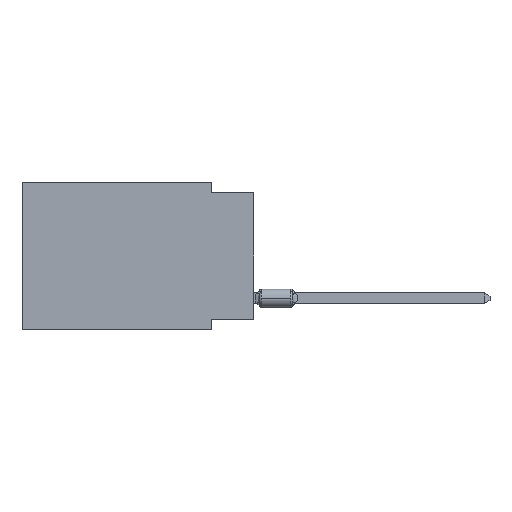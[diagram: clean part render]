
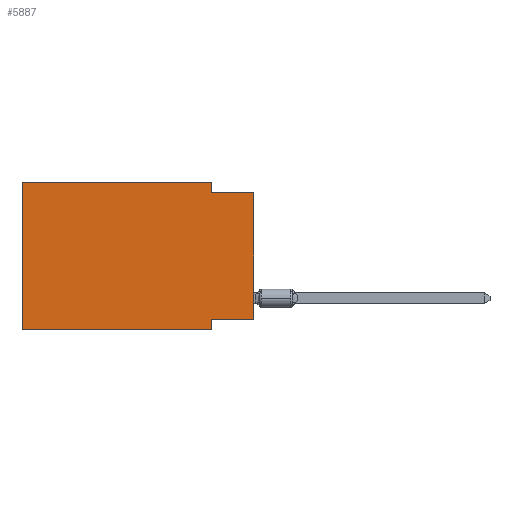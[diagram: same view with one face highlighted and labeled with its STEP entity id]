
A CAD part, left-side view. The second image highlights one B-rep face of the part: STEP entity #5887.
In plain terms, the highlighted planar face has unit normal (-1, 0, 0).
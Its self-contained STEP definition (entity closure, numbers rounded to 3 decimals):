
#1054 = CARTESIAN_POINT ( 'NONE',  ( 0., 0., -8.255 ) ) ;
#1196 = VERTEX_POINT ( 'NONE', #10897 ) ;
#1510 = VERTEX_POINT ( 'NONE', #1054 ) ;
#1604 = EDGE_CURVE ( 'NONE', #11861, #15108, #10876, .T. ) ;
#1928 = VECTOR ( 'NONE', #3988, 1000. ) ;
#2575 = DIRECTION ( 'NONE',  ( 0., 0., -1. ) ) ;
#2758 = ORIENTED_EDGE ( 'NONE', *, *, #11424, .T. ) ;
#3067 = CARTESIAN_POINT ( 'NONE',  ( 0., 0., -8.255 ) ) ;
#3241 = CARTESIAN_POINT ( 'NONE',  ( 0., 2.54, -0.635 ) ) ;
#3458 = DIRECTION ( 'NONE',  ( 0., 0., -1. ) ) ;
#3730 = CARTESIAN_POINT ( 'NONE',  ( 0., 0., -0.635 ) ) ;
#3978 = EDGE_LOOP ( 'NONE', ( #2758, #16378, #6349, #15202, #6863, #8228, #16257, #8611 ) ) ;
#3988 = DIRECTION ( 'NONE',  ( 0., -1., 0. ) ) ;
#4108 = CARTESIAN_POINT ( 'NONE',  ( 0., 2.54, -8.89 ) ) ;
#4757 = VERTEX_POINT ( 'NONE', #3730 ) ;
#4802 = CARTESIAN_POINT ( 'NONE',  ( 0., 2.54, 0. ) ) ;
#5887 = ADVANCED_FACE ( 'NONE', ( #13274 ), #14626, .F. ) ;
#6235 = VECTOR ( 'NONE', #2575, 1000. ) ;
#6247 = VECTOR ( 'NONE', #9762, 1000. ) ;
#6349 = ORIENTED_EDGE ( 'NONE', *, *, #11225, .F. ) ;
#6511 = CARTESIAN_POINT ( 'NONE',  ( 0., 13.97, 0. ) ) ;
#6512 = DIRECTION ( 'NONE',  ( 0., -1., 0. ) ) ;
#6560 = LINE ( 'NONE', #16390, #9378 ) ;
#6678 = CARTESIAN_POINT ( 'NONE',  ( 0., 0., -0.635 ) ) ;
#6863 = ORIENTED_EDGE ( 'NONE', *, *, #12071, .F. ) ;
#7959 = CARTESIAN_POINT ( 'NONE',  ( 0., 13.97, -8.89 ) ) ;
#7978 = VECTOR ( 'NONE', #14712, 1000. ) ;
#8228 = ORIENTED_EDGE ( 'NONE', *, *, #11816, .T. ) ;
#8247 = VERTEX_POINT ( 'NONE', #9148 ) ;
#8556 = DIRECTION ( 'NONE',  ( 0., 1., 0. ) ) ;
#8611 = ORIENTED_EDGE ( 'NONE', *, *, #17129, .F. ) ;
#9148 = CARTESIAN_POINT ( 'NONE',  ( 0., 13.97, -8.89 ) ) ;
#9378 = VECTOR ( 'NONE', #13575, 1000. ) ;
#9762 = DIRECTION ( 'NONE',  ( 0., 0., 1. ) ) ;
#10570 = DIRECTION ( 'NONE',  ( 1., 0., 0. ) ) ;
#10571 = LINE ( 'NONE', #7959, #7978 ) ;
#10876 = LINE ( 'NONE', #4108, #6235 ) ;
#10897 = CARTESIAN_POINT ( 'NONE',  ( 0., 2.54, 0. ) ) ;
#11225 = EDGE_CURVE ( 'NONE', #1196, #15140, #17165, .T. ) ;
#11424 = EDGE_CURVE ( 'NONE', #1510, #4757, #15188, .T. ) ;
#11715 = EDGE_CURVE ( 'NONE', #15140, #4757, #16080, .T. ) ;
#11734 = EDGE_CURVE ( 'NONE', #14815, #1196, #17601, .T. ) ;
#11816 = EDGE_CURVE ( 'NONE', #8247, #15108, #10571, .T. ) ;
#11861 = VERTEX_POINT ( 'NONE', #15253 ) ;
#12071 = EDGE_CURVE ( 'NONE', #8247, #14815, #6560, .T. ) ;
#12311 = CARTESIAN_POINT ( 'NONE',  ( 0., 0., 0. ) ) ;
#12433 = AXIS2_PLACEMENT_3D ( 'NONE', #6511, #10570, #14711 ) ;
#13274 = FACE_OUTER_BOUND ( 'NONE', #3978, .T. ) ;
#13408 = VECTOR ( 'NONE', #8556, 1000. ) ;
#13575 = DIRECTION ( 'NONE',  ( 0., 0., 1. ) ) ;
#13970 = CARTESIAN_POINT ( 'NONE',  ( 0., 2.54, -8.89 ) ) ;
#14248 = CARTESIAN_POINT ( 'NONE',  ( 0., 13.97, 0. ) ) ;
#14626 = PLANE ( 'NONE',  #12433 ) ;
#14711 = DIRECTION ( 'NONE',  ( 0., 0., -1. ) ) ;
#14712 = DIRECTION ( 'NONE',  ( 0., -1., 0. ) ) ;
#14799 = CARTESIAN_POINT ( 'NONE',  ( 0., 13.97, 0. ) ) ;
#14815 = VERTEX_POINT ( 'NONE', #14248 ) ;
#15108 = VERTEX_POINT ( 'NONE', #13970 ) ;
#15140 = VERTEX_POINT ( 'NONE', #3241 ) ;
#15188 = LINE ( 'NONE', #12311, #6247 ) ;
#15202 = ORIENTED_EDGE ( 'NONE', *, *, #11734, .F. ) ;
#15253 = CARTESIAN_POINT ( 'NONE',  ( 0., 2.54, -8.255 ) ) ;
#16080 = LINE ( 'NONE', #6678, #1928 ) ;
#16257 = ORIENTED_EDGE ( 'NONE', *, *, #1604, .F. ) ;
#16378 = ORIENTED_EDGE ( 'NONE', *, *, #11715, .F. ) ;
#16390 = CARTESIAN_POINT ( 'NONE',  ( 0., 13.97, 0. ) ) ;
#16599 = VECTOR ( 'NONE', #3458, 1000. ) ;
#16755 = LINE ( 'NONE', #3067, #13408 ) ;
#17129 = EDGE_CURVE ( 'NONE', #1510, #11861, #16755, .T. ) ;
#17165 = LINE ( 'NONE', #4802, #16599 ) ;
#17479 = VECTOR ( 'NONE', #6512, 1000. ) ;
#17601 = LINE ( 'NONE', #14799, #17479 ) ;
